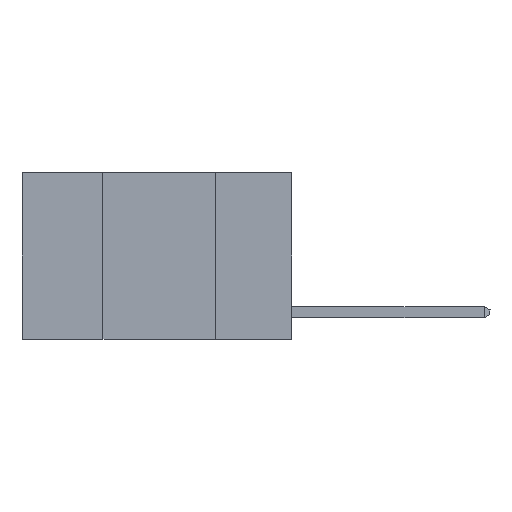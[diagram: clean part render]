
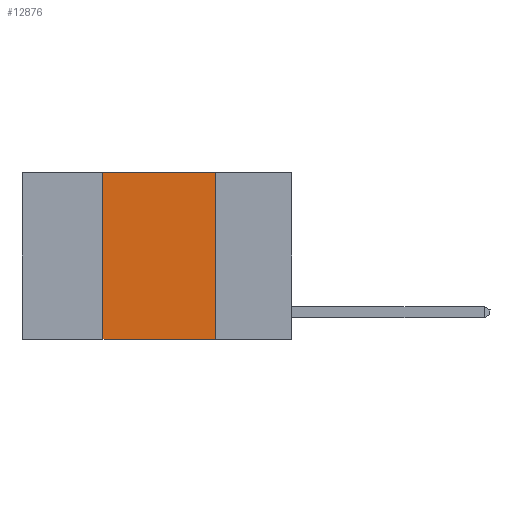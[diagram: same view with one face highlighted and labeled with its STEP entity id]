
A CAD part, left-side view. The second image highlights one B-rep face of the part: STEP entity #12876.
In plain terms, the highlighted planar face has unit normal (-1, 0, 0).
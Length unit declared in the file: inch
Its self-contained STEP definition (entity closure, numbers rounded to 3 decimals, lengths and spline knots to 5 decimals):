
#18 = DIRECTION ( 'NONE',  ( 1., 0., 0. ) ) ;
#158 = VERTEX_POINT ( 'NONE', #4654 ) ;
#262 = CARTESIAN_POINT ( 'NONE',  ( 0., 0.42, -0.37 ) ) ;
#299 = AXIS2_PLACEMENT_3D ( 'NONE', #7111, #18, #8262 ) ;
#335 = DIRECTION ( 'NONE',  ( 0., 0., 1. ) ) ;
#961 = EDGE_LOOP ( 'NONE', ( #13119, #14189, #2278, #3016 ) ) ;
#1470 = FACE_OUTER_BOUND ( 'NONE', #961, .T. ) ;
#2006 = CARTESIAN_POINT ( 'NONE',  ( 0., 0.6, -0.37 ) ) ;
#2278 = ORIENTED_EDGE ( 'NONE', *, *, #13306, .F. ) ;
#2314 = EDGE_CURVE ( 'NONE', #3357, #6861, #8356, .T. ) ;
#2421 = VECTOR ( 'NONE', #5375, 39.37008 ) ;
#3016 = ORIENTED_EDGE ( 'NONE', *, *, #2314, .T. ) ;
#3191 = DIRECTION ( 'NONE',  ( 0., -1., 0. ) ) ;
#3357 = VERTEX_POINT ( 'NONE', #262 ) ;
#4215 = CARTESIAN_POINT ( 'NONE',  ( 0., 0.17, 0. ) ) ;
#4654 = CARTESIAN_POINT ( 'NONE',  ( 0., 0.17, 0. ) ) ;
#4795 = CARTESIAN_POINT ( 'NONE',  ( 0., 0.6, 0. ) ) ;
#5061 = CARTESIAN_POINT ( 'NONE',  ( 0., 0.42, 0. ) ) ;
#5375 = DIRECTION ( 'NONE',  ( 0., 0., -1. ) ) ;
#6861 = VERTEX_POINT ( 'NONE', #7097 ) ;
#7097 = CARTESIAN_POINT ( 'NONE',  ( 0., 0.17, -0.37 ) ) ;
#7111 = CARTESIAN_POINT ( 'NONE',  ( 0., 0.6, 0. ) ) ;
#7299 = VERTEX_POINT ( 'NONE', #10000 ) ;
#7606 = EDGE_CURVE ( 'NONE', #7299, #158, #10586, .T. ) ;
#7992 = VECTOR ( 'NONE', #3191, 39.37008 ) ;
#8262 = DIRECTION ( 'NONE',  ( 0., 0., -1. ) ) ;
#8356 = LINE ( 'NONE', #2006, #7992 ) ;
#8600 = LINE ( 'NONE', #4215, #2421 ) ;
#9526 = VECTOR ( 'NONE', #335, 39.37008 ) ;
#10000 = CARTESIAN_POINT ( 'NONE',  ( 0., 0.42, 0. ) ) ;
#10586 = LINE ( 'NONE', #4795, #13956 ) ;
#12561 = LINE ( 'NONE', #5061, #9526 ) ;
#12565 = EDGE_CURVE ( 'NONE', #158, #6861, #8600, .T. ) ;
#12876 = ADVANCED_FACE ( 'NONE', ( #1470 ), #13975, .F. ) ;
#12884 = DIRECTION ( 'NONE',  ( 0., -1., 0. ) ) ;
#13119 = ORIENTED_EDGE ( 'NONE', *, *, #12565, .F. ) ;
#13306 = EDGE_CURVE ( 'NONE', #3357, #7299, #12561, .T. ) ;
#13956 = VECTOR ( 'NONE', #12884, 39.37008 ) ;
#13975 = PLANE ( 'NONE',  #299 ) ;
#14189 = ORIENTED_EDGE ( 'NONE', *, *, #7606, .F. ) ;
